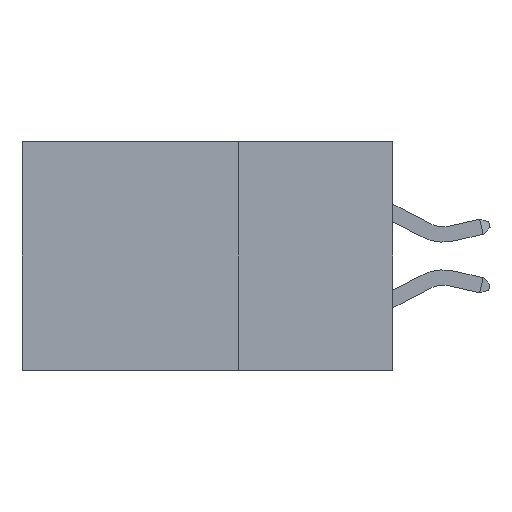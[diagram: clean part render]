
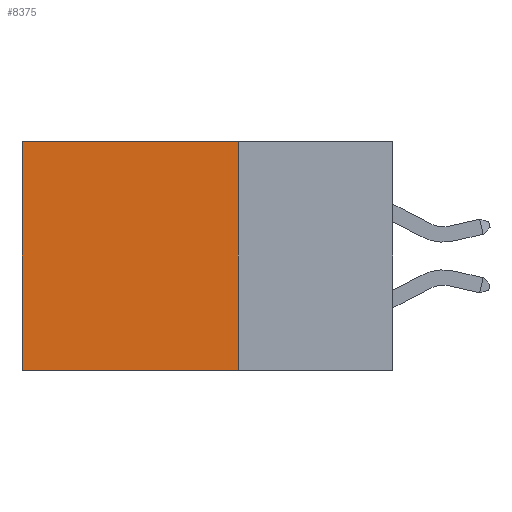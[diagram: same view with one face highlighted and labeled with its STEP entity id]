
A CAD part, left-side view. The second image highlights one B-rep face of the part: STEP entity #8375.
In plain terms, the highlighted planar face has unit normal (-1, 0, 0).
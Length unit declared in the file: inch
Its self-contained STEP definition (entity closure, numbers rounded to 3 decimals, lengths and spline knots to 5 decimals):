
#151 = DIRECTION ( 'NONE',  ( 0., 0., -1. ) ) ;
#963 = EDGE_CURVE ( 'NONE', #16695, #19891, #12320, .T. ) ;
#1213 = FACE_OUTER_BOUND ( 'NONE', #1819, .T. ) ;
#1470 = LINE ( 'NONE', #18425, #3880 ) ;
#1819 = EDGE_LOOP ( 'NONE', ( #19928, #27747, #28897, #27235 ) ) ;
#3112 = VECTOR ( 'NONE', #6837, 39.37008 ) ;
#3880 = VECTOR ( 'NONE', #27539, 39.37008 ) ;
#6172 = VECTOR ( 'NONE', #28894, 39.37008 ) ;
#6313 = EDGE_CURVE ( 'NONE', #21671, #19891, #19022, .T. ) ;
#6837 = DIRECTION ( 'NONE',  ( 0., 1., 0. ) ) ;
#6988 = CARTESIAN_POINT ( 'NONE',  ( 0.2875, 0.25, -0.37 ) ) ;
#8150 = AXIS2_PLACEMENT_3D ( 'NONE', #18178, #11099, #10643 ) ;
#8375 = ADVANCED_FACE ( 'NONE', ( #1213 ), #25239, .F. ) ;
#10643 = DIRECTION ( 'NONE',  ( 0., 0., -1. ) ) ;
#10937 = CARTESIAN_POINT ( 'NONE',  ( 0.2875, 0.6, -0.37 ) ) ;
#11099 = DIRECTION ( 'NONE',  ( 1., 0., 0. ) ) ;
#12320 = LINE ( 'NONE', #19575, #3112 ) ;
#13841 = EDGE_CURVE ( 'NONE', #19444, #21671, #1470, .T. ) ;
#16331 = CARTESIAN_POINT ( 'NONE',  ( 0.2875, 0.25, 0. ) ) ;
#16695 = VERTEX_POINT ( 'NONE', #6988 ) ;
#18178 = CARTESIAN_POINT ( 'NONE',  ( 0.2875, 0.25, 0. ) ) ;
#18425 = CARTESIAN_POINT ( 'NONE',  ( 0.2875, 0.25, 0. ) ) ;
#18788 = VECTOR ( 'NONE', #151, 39.37008 ) ;
#19022 = LINE ( 'NONE', #21838, #6172 ) ;
#19444 = VERTEX_POINT ( 'NONE', #23219 ) ;
#19575 = CARTESIAN_POINT ( 'NONE',  ( 0.2875, 0.25, -0.37 ) ) ;
#19687 = CARTESIAN_POINT ( 'NONE',  ( 0.2875, 0.6, 0. ) ) ;
#19891 = VERTEX_POINT ( 'NONE', #10937 ) ;
#19928 = ORIENTED_EDGE ( 'NONE', *, *, #6313, .T. ) ;
#21200 = LINE ( 'NONE', #16331, #18788 ) ;
#21671 = VERTEX_POINT ( 'NONE', #19687 ) ;
#21838 = CARTESIAN_POINT ( 'NONE',  ( 0.2875, 0.6, 0. ) ) ;
#23219 = CARTESIAN_POINT ( 'NONE',  ( 0.2875, 0.25, 0. ) ) ;
#25239 = PLANE ( 'NONE',  #8150 ) ;
#27235 = ORIENTED_EDGE ( 'NONE', *, *, #13841, .T. ) ;
#27539 = DIRECTION ( 'NONE',  ( 0., 1., 0. ) ) ;
#27542 = EDGE_CURVE ( 'NONE', #19444, #16695, #21200, .T. ) ;
#27747 = ORIENTED_EDGE ( 'NONE', *, *, #963, .F. ) ;
#28894 = DIRECTION ( 'NONE',  ( 0., 0., -1. ) ) ;
#28897 = ORIENTED_EDGE ( 'NONE', *, *, #27542, .F. ) ;
